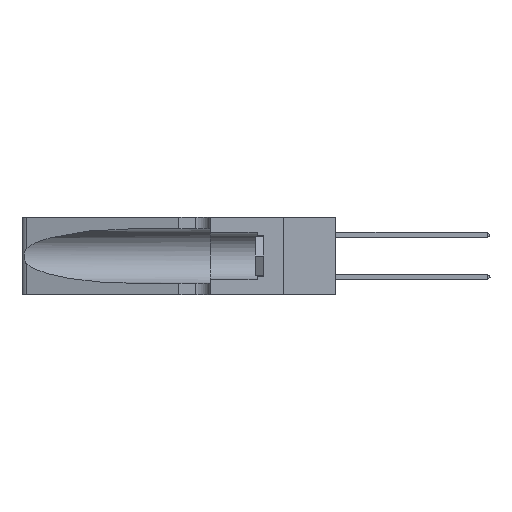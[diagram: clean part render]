
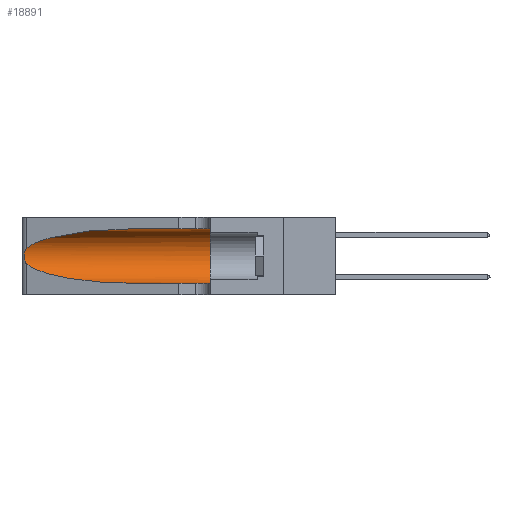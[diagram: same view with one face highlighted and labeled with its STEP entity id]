
A CAD part, left-side view. The second image highlights one B-rep face of the part: STEP entity #18891.
In plain terms, the highlighted cylindrical face has radius 3.308 mm (diameter 6.617 mm), a partial arc.
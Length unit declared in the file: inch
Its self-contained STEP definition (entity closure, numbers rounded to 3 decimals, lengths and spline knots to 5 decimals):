
#48 = CARTESIAN_POINT ( 'NONE',  ( 0.18966, 0.96281, 0.31525 ) ) ;
#530 = CYLINDRICAL_SURFACE ( 'NONE', #1361, 0.13025 ) ;
#831 = EDGE_CURVE ( 'NONE', #6373, #4716, #7008, .T. ) ;
#1361 = AXIS2_PLACEMENT_3D ( 'NONE', #26430, #28511, #13026 ) ;
#1793 = DIRECTION ( 'NONE',  ( 0., 1., 0. ) ) ;
#1940 = CARTESIAN_POINT ( 'NONE',  ( 0.25487, 1.22718, 0.14631 ) ) ;
#3061 = CARTESIAN_POINT ( 'NONE',  ( 0.25487, 1.22718, 0.22369 ) ) ;
#3203 = VERTEX_POINT ( 'NONE', #12475 ) ;
#4453 = DIRECTION ( 'NONE',  ( 0., 0., 1. ) ) ;
#4464 = CARTESIAN_POINT ( 'NONE',  ( 0.25555, 1.22993, 0.14849 ) ) ;
#4716 = VERTEX_POINT ( 'NONE', #21968 ) ;
#4829 = CARTESIAN_POINT ( 'NONE',  ( 0.18966, 0.96281, 0.05475 ) ) ;
#5094 = DIRECTION ( 'NONE',  ( 0., -1., 0. ) ) ;
#5310 = CARTESIAN_POINT ( 'NONE',  ( 0.1305, 0.72297, 0.31525 ) ) ;
#6373 = VERTEX_POINT ( 'NONE', #3061 ) ;
#6628 = CARTESIAN_POINT ( 'NONE',  ( 0.1305, 0.72297, 0.05475 ) ) ;
#7008 = B_SPLINE_CURVE_WITH_KNOTS ( 'NONE', 3,
 ( #27451, #9661, #30262, #30394, #11701, #16527, #27098, #17993, #30552, #17902, #20495, #15309, #4464, #1940 ),
 .UNSPECIFIED., .F., .F.,
 ( 4, 2, 2, 2, 2, 2, 4 ),
 ( 0., 0.00027, 0.00053, 0.00107, 0.0016, 0.00187, 0.00214 ),
 .UNSPECIFIED. ) ;
#7450 = AXIS2_PLACEMENT_3D ( 'NONE', #14826, #1793, #4453 ) ;
#8342 = VERTEX_POINT ( 'NONE', #28059 ) ;
#9231 = VECTOR ( 'NONE', #5094, 39.37008 ) ;
#9365 = EDGE_CURVE ( 'NONE', #33469, #8342, #28638, .T. ) ;
#9645 = ORIENTED_EDGE ( 'NONE', *, *, #831, .T. ) ;
#9661 = CARTESIAN_POINT ( 'NONE',  ( 0.25555, 1.22994, 0.2215 ) ) ;
#9971 =( BOUNDED_CURVE ( )  B_SPLINE_CURVE ( 3, ( #5310, #48, #10667, #33483 ),
 .UNSPECIFIED., .F., .F. ) 
 B_SPLINE_CURVE_WITH_KNOTS ( ( 4, 4 ),
 ( 1.5708, 2.84003 ),
 .UNSPECIFIED. ) 
 CURVE ( )  GEOMETRIC_REPRESENTATION_ITEM ( )  RATIONAL_B_SPLINE_CURVE ( ( 1., 0.87, 0.87, 1. ) ) 
 REPRESENTATION_ITEM ( '' )  );
#10275 = ORIENTED_EDGE ( 'NONE', *, *, #9365, .T. ) ;
#10667 = CARTESIAN_POINT ( 'NONE',  ( 0.2373, 1.15595, 0.28018 ) ) ;
#11701 = CARTESIAN_POINT ( 'NONE',  ( 0.25854, 1.2359, 0.20912 ) ) ;
#12094 = CARTESIAN_POINT ( 'NONE',  ( 0.1305, 1.61858, 0.05475 ) ) ;
#12475 = CARTESIAN_POINT ( 'NONE',  ( 0.1305, 0.72297, 0.31525 ) ) ;
#12922 = FACE_OUTER_BOUND ( 'NONE', #29697, .T. ) ;
#13026 = DIRECTION ( 'NONE',  ( 0., 0., -1. ) ) ;
#13033 = CARTESIAN_POINT ( 'NONE',  ( 0.25487, 1.22718, 0.14631 ) ) ;
#14101 = CARTESIAN_POINT ( 'NONE',  ( 0.1305, 0.35, 0.31525 ) ) ;
#14826 = CARTESIAN_POINT ( 'NONE',  ( 0.1305, 0.35, 0.185 ) ) ;
#15309 = CARTESIAN_POINT ( 'NONE',  ( 0.25639, 1.23186, 0.15144 ) ) ;
#16486 = LINE ( 'NONE', #28130, #9231 ) ;
#16499 = CIRCLE ( 'NONE', #7450, 0.13025 ) ;
#16527 = CARTESIAN_POINT ( 'NONE',  ( 0.26018, 1.23835, 0.19895 ) ) ;
#17902 = CARTESIAN_POINT ( 'NONE',  ( 0.25856, 1.23593, 0.16098 ) ) ;
#17993 = CARTESIAN_POINT ( 'NONE',  ( 0.26075, 1.23896, 0.178 ) ) ;
#18373 = VERTEX_POINT ( 'NONE', #14101 ) ;
#18891 = ADVANCED_FACE ( 'NONE', ( #12922 ), #530, .F. ) ;
#19439 =( BOUNDED_CURVE ( )  B_SPLINE_CURVE ( 3, ( #13033, #31141, #4829, #28717 ),
 .UNSPECIFIED., .F., .F. ) 
 B_SPLINE_CURVE_WITH_KNOTS ( ( 4, 4 ),
 ( 3.44316, 4.71239 ),
 .UNSPECIFIED. ) 
 CURVE ( )  GEOMETRIC_REPRESENTATION_ITEM ( )  RATIONAL_B_SPLINE_CURVE ( ( 1., 0.87, 0.87, 1. ) ) 
 REPRESENTATION_ITEM ( '' )  );
#20495 = CARTESIAN_POINT ( 'NONE',  ( 0.25789, 1.23486, 0.15765 ) ) ;
#21968 = CARTESIAN_POINT ( 'NONE',  ( 0.25487, 1.22718, 0.14631 ) ) ;
#22252 = EDGE_CURVE ( 'NONE', #3203, #6373, #9971, .T. ) ;
#24070 = EDGE_CURVE ( 'NONE', #3203, #18373, #16486, .T. ) ;
#24569 = VECTOR ( 'NONE', #32987, 39.37008 ) ;
#24845 = ORIENTED_EDGE ( 'NONE', *, *, #22252, .T. ) ;
#25091 = ORIENTED_EDGE ( 'NONE', *, *, #32861, .T. ) ;
#26210 = ORIENTED_EDGE ( 'NONE', *, *, #24070, .F. ) ;
#26430 = CARTESIAN_POINT ( 'NONE',  ( 0.1305, 1.61858, 0.185 ) ) ;
#27098 = CARTESIAN_POINT ( 'NONE',  ( 0.26075, 1.23896, 0.19203 ) ) ;
#27451 = CARTESIAN_POINT ( 'NONE',  ( 0.25487, 1.22718, 0.22369 ) ) ;
#28059 = CARTESIAN_POINT ( 'NONE',  ( 0.1305, 0.35, 0.05475 ) ) ;
#28130 = CARTESIAN_POINT ( 'NONE',  ( 0.1305, 1.61858, 0.31525 ) ) ;
#28511 = DIRECTION ( 'NONE',  ( 0., -1., 0. ) ) ;
#28638 = LINE ( 'NONE', #12094, #24569 ) ;
#28717 = CARTESIAN_POINT ( 'NONE',  ( 0.1305, 0.72297, 0.05475 ) ) ;
#28940 = EDGE_CURVE ( 'NONE', #18373, #8342, #16499, .T. ) ;
#29697 = EDGE_LOOP ( 'NONE', ( #24845, #9645, #25091, #10275, #33167, #26210 ) ) ;
#30262 = CARTESIAN_POINT ( 'NONE',  ( 0.25639, 1.23184, 0.21858 ) ) ;
#30394 = CARTESIAN_POINT ( 'NONE',  ( 0.25787, 1.23484, 0.2124 ) ) ;
#30552 = CARTESIAN_POINT ( 'NONE',  ( 0.26017, 1.23833, 0.17102 ) ) ;
#31141 = CARTESIAN_POINT ( 'NONE',  ( 0.2373, 1.15595, 0.08982 ) ) ;
#32861 = EDGE_CURVE ( 'NONE', #4716, #33469, #19439, .T. ) ;
#32987 = DIRECTION ( 'NONE',  ( 0., -1., 0. ) ) ;
#33167 = ORIENTED_EDGE ( 'NONE', *, *, #28940, .F. ) ;
#33469 = VERTEX_POINT ( 'NONE', #6628 ) ;
#33483 = CARTESIAN_POINT ( 'NONE',  ( 0.25487, 1.22718, 0.22369 ) ) ;
